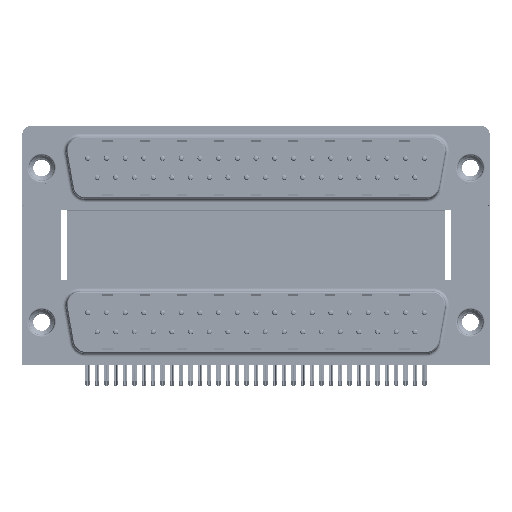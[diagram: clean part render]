
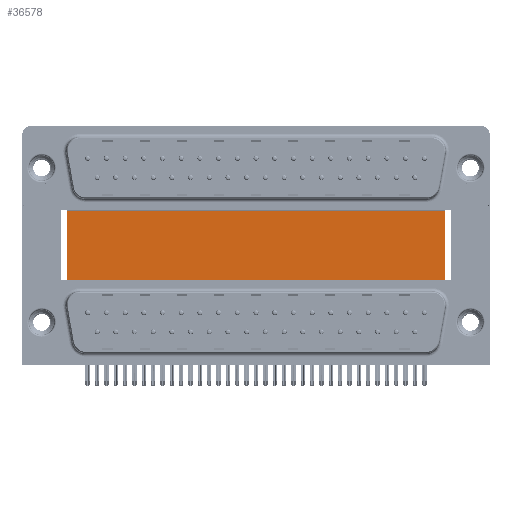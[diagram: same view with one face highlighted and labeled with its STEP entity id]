
A CAD part, top view. The second image highlights one B-rep face of the part: STEP entity #36578.
In plain terms, the highlighted planar face has unit normal (0, 0, 1).
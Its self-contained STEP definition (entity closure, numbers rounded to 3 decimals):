
#151 = DIRECTION ( 'NONE',  ( 1., 0., 0. ) ) ;
#1375 = LINE ( 'NONE', #26437, #42444 ) ;
#4952 = EDGE_LOOP ( 'NONE', ( #48481, #19052, #52684, #31785 ) ) ;
#5014 = VERTEX_POINT ( 'NONE', #32220 ) ;
#7027 = DIRECTION ( 'NONE',  ( 0., -1., 0. ) ) ;
#7142 = CARTESIAN_POINT ( 'NONE',  ( 3.79, 16.585, -12. ) ) ;
#8972 = VECTOR ( 'NONE', #18224, 1000. ) ;
#9006 = AXIS2_PLACEMENT_3D ( 'NONE', #49235, #12257, #40587 ) ;
#11729 = PLANE ( 'NONE',  #9006 ) ;
#12257 = DIRECTION ( 'NONE',  ( 0., 0., -1. ) ) ;
#12920 = EDGE_CURVE ( 'NONE', #5014, #22803, #52487, .T. ) ;
#13792 = LINE ( 'NONE', #30243, #17857 ) ;
#15524 = CARTESIAN_POINT ( 'NONE',  ( 3.79, -3.735, -12. ) ) ;
#15529 = CARTESIAN_POINT ( 'NONE',  ( 59.71, -3.735, -12. ) ) ;
#17857 = VECTOR ( 'NONE', #7027, 1000. ) ;
#18224 = DIRECTION ( 'NONE',  ( 1., 0., 0. ) ) ;
#19052 = ORIENTED_EDGE ( 'NONE', *, *, #42200, .F. ) ;
#22788 = LINE ( 'NONE', #7142, #8972 ) ;
#22803 = VERTEX_POINT ( 'NONE', #15529 ) ;
#22902 = DIRECTION ( 'NONE',  ( 0., -1., 0. ) ) ;
#26437 = CARTESIAN_POINT ( 'NONE',  ( 3.79, 16.585, -12. ) ) ;
#30243 = CARTESIAN_POINT ( 'NONE',  ( 59.71, 16.585, -12. ) ) ;
#31689 = CARTESIAN_POINT ( 'NONE',  ( 3.79, 16.585, -12. ) ) ;
#31785 = ORIENTED_EDGE ( 'NONE', *, *, #45933, .T. ) ;
#32220 = CARTESIAN_POINT ( 'NONE',  ( 3.79, -3.735, -12. ) ) ;
#36457 = EDGE_CURVE ( 'NONE', #43145, #49993, #22788, .T. ) ;
#36578 = ADVANCED_FACE ( 'NONE', ( #48970 ), #11729, .F. ) ;
#36709 = CARTESIAN_POINT ( 'NONE',  ( 59.71, 16.585, -12. ) ) ;
#40587 = DIRECTION ( 'NONE',  ( -1., 0., 0. ) ) ;
#42200 = EDGE_CURVE ( 'NONE', #49993, #22803, #13792, .T. ) ;
#42444 = VECTOR ( 'NONE', #22902, 1000. ) ;
#43145 = VERTEX_POINT ( 'NONE', #31689 ) ;
#45933 = EDGE_CURVE ( 'NONE', #43145, #5014, #1375, .T. ) ;
#48481 = ORIENTED_EDGE ( 'NONE', *, *, #12920, .T. ) ;
#48970 = FACE_OUTER_BOUND ( 'NONE', #4952, .T. ) ;
#49235 = CARTESIAN_POINT ( 'NONE',  ( 3.79, 16.585, -12. ) ) ;
#49993 = VERTEX_POINT ( 'NONE', #36709 ) ;
#50914 = VECTOR ( 'NONE', #151, 1000. ) ;
#52487 = LINE ( 'NONE', #15524, #50914 ) ;
#52684 = ORIENTED_EDGE ( 'NONE', *, *, #36457, .F. ) ;
